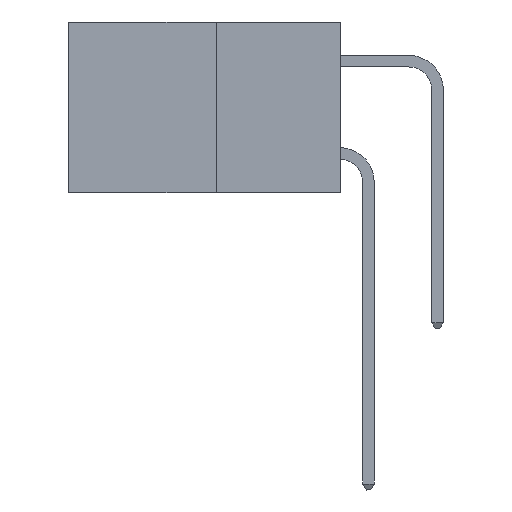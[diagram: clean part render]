
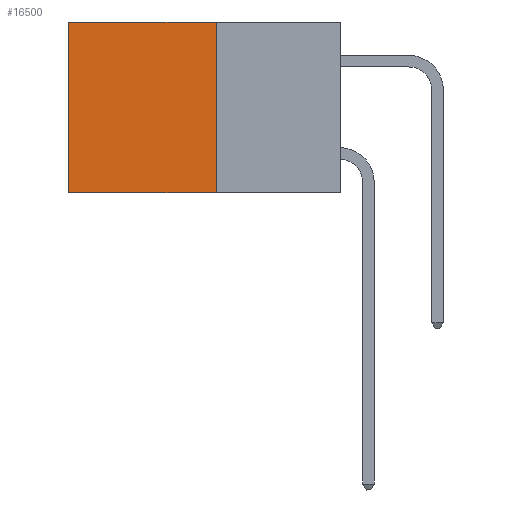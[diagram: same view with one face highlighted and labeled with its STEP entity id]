
A CAD part, left-side view. The second image highlights one B-rep face of the part: STEP entity #16500.
In plain terms, the highlighted planar face has unit normal (-1, 0, 0).
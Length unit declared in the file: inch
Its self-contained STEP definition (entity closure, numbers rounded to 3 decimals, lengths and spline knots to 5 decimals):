
#92 = EDGE_CURVE ( 'NONE', #15396, #5226, #19770, .T. ) ;
#419 = ORIENTED_EDGE ( 'NONE', *, *, #2356, .T. ) ;
#1811 = DIRECTION ( 'NONE',  ( 0., 0., -1. ) ) ;
#2356 = EDGE_CURVE ( 'NONE', #14128, #18623, #10502, .T. ) ;
#4147 = DIRECTION ( 'NONE',  ( 0., 0., -1. ) ) ;
#4693 = CARTESIAN_POINT ( 'NONE',  ( 0.277, 0.27, 0. ) ) ;
#4873 = ORIENTED_EDGE ( 'NONE', *, *, #14333, .T. ) ;
#5226 = VERTEX_POINT ( 'NONE', #15599 ) ;
#5727 = VECTOR ( 'NONE', #12513, 39.37008 ) ;
#6700 = DIRECTION ( 'NONE',  ( 0., 1., 0. ) ) ;
#7290 = VECTOR ( 'NONE', #1811, 39.37008 ) ;
#7426 = CARTESIAN_POINT ( 'NONE',  ( 0.277, 0.27, -0.37 ) ) ;
#7954 = CARTESIAN_POINT ( 'NONE',  ( 0.277, 0.27, -0.37 ) ) ;
#8892 = AXIS2_PLACEMENT_3D ( 'NONE', #7426, #13821, #4147 ) ;
#10386 = CARTESIAN_POINT ( 'NONE',  ( 0.277, 0.59, -0.37 ) ) ;
#10502 = LINE ( 'NONE', #10386, #17780 ) ;
#11835 = EDGE_LOOP ( 'NONE', ( #419, #12046, #15878, #4873 ) ) ;
#12046 = ORIENTED_EDGE ( 'NONE', *, *, #12908, .F. ) ;
#12193 = CARTESIAN_POINT ( 'NONE',  ( 0.277, 0.59, 0. ) ) ;
#12513 = DIRECTION ( 'NONE',  ( 0., 1., 0. ) ) ;
#12908 = EDGE_CURVE ( 'NONE', #5226, #18623, #15215, .T. ) ;
#13821 = DIRECTION ( 'NONE',  ( 1., 0., 0. ) ) ;
#14067 = CARTESIAN_POINT ( 'NONE',  ( 0.277, 0.27, -0.37 ) ) ;
#14128 = VERTEX_POINT ( 'NONE', #12193 ) ;
#14333 = EDGE_CURVE ( 'NONE', #15396, #14128, #16382, .T. ) ;
#14361 = DIRECTION ( 'NONE',  ( 0., 0., -1. ) ) ;
#15215 = LINE ( 'NONE', #14067, #5727 ) ;
#15396 = VERTEX_POINT ( 'NONE', #4693 ) ;
#15599 = CARTESIAN_POINT ( 'NONE',  ( 0.277, 0.27, -0.37 ) ) ;
#15878 = ORIENTED_EDGE ( 'NONE', *, *, #92, .F. ) ;
#16382 = LINE ( 'NONE', #19176, #19941 ) ;
#16500 = ADVANCED_FACE ( 'NONE', ( #17054 ), #19867, .F. ) ;
#17054 = FACE_OUTER_BOUND ( 'NONE', #11835, .T. ) ;
#17780 = VECTOR ( 'NONE', #14361, 39.37008 ) ;
#18408 = CARTESIAN_POINT ( 'NONE',  ( 0.277, 0.59, -0.37 ) ) ;
#18623 = VERTEX_POINT ( 'NONE', #18408 ) ;
#19176 = CARTESIAN_POINT ( 'NONE',  ( 0.277, 0.27, 0. ) ) ;
#19770 = LINE ( 'NONE', #7954, #7290 ) ;
#19867 = PLANE ( 'NONE',  #8892 ) ;
#19941 = VECTOR ( 'NONE', #6700, 39.37008 ) ;
